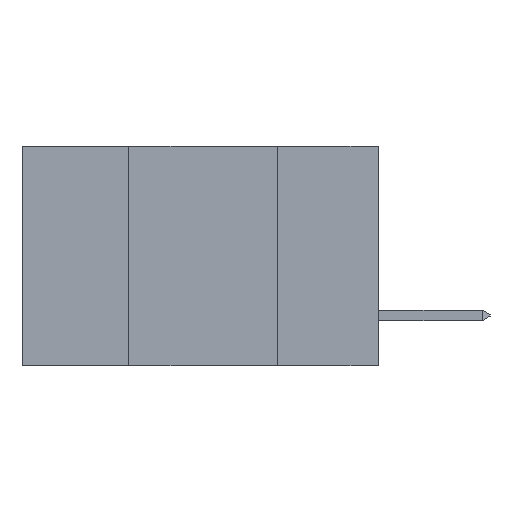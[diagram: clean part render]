
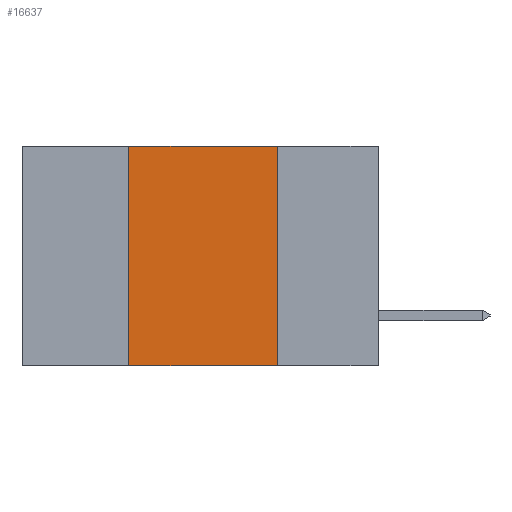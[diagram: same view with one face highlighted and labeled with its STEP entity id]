
A CAD part, left-side view. The second image highlights one B-rep face of the part: STEP entity #16637.
In plain terms, the highlighted planar face has unit normal (-1, 0, 0).
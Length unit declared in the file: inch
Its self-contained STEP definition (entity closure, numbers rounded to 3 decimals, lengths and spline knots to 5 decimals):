
#17 = EDGE_CURVE ( 'NONE', #11303, #8185, #5371, .T. ) ;
#49 = VECTOR ( 'NONE', #23160, 39.37008 ) ;
#393 = ORIENTED_EDGE ( 'NONE', *, *, #16137, .T. ) ;
#443 = DIRECTION ( 'NONE',  ( 0., -1., 0. ) ) ;
#1097 = CARTESIAN_POINT ( 'NONE',  ( 0., 0.42, 0. ) ) ;
#2154 = VERTEX_POINT ( 'NONE', #12902 ) ;
#3093 = DIRECTION ( 'NONE',  ( 0., 0., 1. ) ) ;
#3681 = EDGE_CURVE ( 'NONE', #8185, #8079, #9183, .T. ) ;
#4053 = LINE ( 'NONE', #1097, #24184 ) ;
#4309 = CARTESIAN_POINT ( 'NONE',  ( 0., 0.6, 0. ) ) ;
#5371 = LINE ( 'NONE', #4309, #49 ) ;
#5864 = CARTESIAN_POINT ( 'NONE',  ( 0., 0.6, 0. ) ) ;
#6198 = CARTESIAN_POINT ( 'NONE',  ( 0., 0.17, -0.37 ) ) ;
#7794 = CARTESIAN_POINT ( 'NONE',  ( 0., 0.17, 0. ) ) ;
#7838 = DIRECTION ( 'NONE',  ( 0., 0., -1. ) ) ;
#8079 = VERTEX_POINT ( 'NONE', #6198 ) ;
#8185 = VERTEX_POINT ( 'NONE', #12441 ) ;
#9183 = LINE ( 'NONE', #7794, #23426 ) ;
#9536 = CARTESIAN_POINT ( 'NONE',  ( 0., 0.42, 0. ) ) ;
#9746 = ORIENTED_EDGE ( 'NONE', *, *, #17, .F. ) ;
#11303 = VERTEX_POINT ( 'NONE', #9536 ) ;
#12441 = CARTESIAN_POINT ( 'NONE',  ( 0., 0.17, 0. ) ) ;
#12902 = CARTESIAN_POINT ( 'NONE',  ( 0., 0.42, -0.37 ) ) ;
#14678 = EDGE_LOOP ( 'NONE', ( #24258, #9746, #14990, #393 ) ) ;
#14990 = ORIENTED_EDGE ( 'NONE', *, *, #21772, .F. ) ;
#15661 = PLANE ( 'NONE',  #16999 ) ;
#16137 = EDGE_CURVE ( 'NONE', #2154, #8079, #23180, .T. ) ;
#16637 = ADVANCED_FACE ( 'NONE', ( #24509 ), #15661, .F. ) ;
#16999 = AXIS2_PLACEMENT_3D ( 'NONE', #5864, #19506, #7838 ) ;
#17549 = DIRECTION ( 'NONE',  ( 0., 0., -1. ) ) ;
#18668 = VECTOR ( 'NONE', #443, 39.37008 ) ;
#19506 = DIRECTION ( 'NONE',  ( 1., 0., 0. ) ) ;
#21772 = EDGE_CURVE ( 'NONE', #2154, #11303, #4053, .T. ) ;
#23160 = DIRECTION ( 'NONE',  ( 0., -1., 0. ) ) ;
#23180 = LINE ( 'NONE', #23904, #18668 ) ;
#23426 = VECTOR ( 'NONE', #17549, 39.37008 ) ;
#23904 = CARTESIAN_POINT ( 'NONE',  ( 0., 0.6, -0.37 ) ) ;
#24184 = VECTOR ( 'NONE', #3093, 39.37008 ) ;
#24258 = ORIENTED_EDGE ( 'NONE', *, *, #3681, .F. ) ;
#24509 = FACE_OUTER_BOUND ( 'NONE', #14678, .T. ) ;
